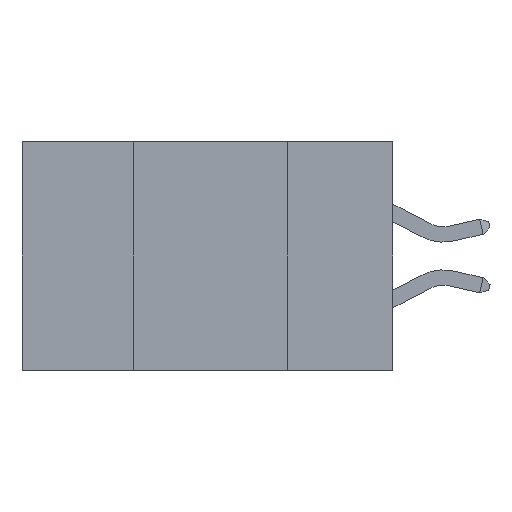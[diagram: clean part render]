
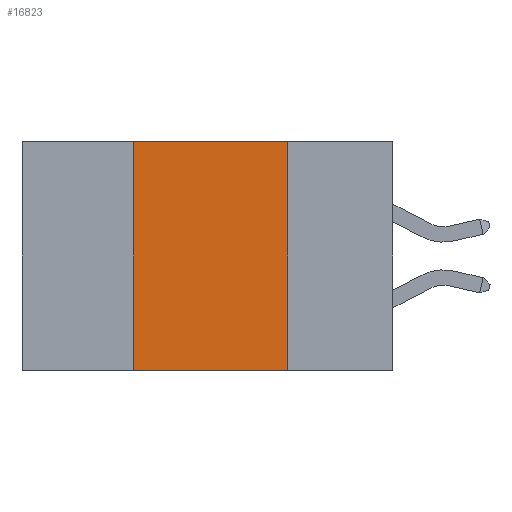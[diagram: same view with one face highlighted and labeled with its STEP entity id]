
A CAD part, left-side view. The second image highlights one B-rep face of the part: STEP entity #16823.
In plain terms, the highlighted planar face has unit normal (-1, 0, 0).
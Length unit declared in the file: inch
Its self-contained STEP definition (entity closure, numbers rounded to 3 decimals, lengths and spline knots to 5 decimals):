
#85 = EDGE_CURVE ( 'NONE', #16612, #15802, #24296, .T. ) ;
#560 = CARTESIAN_POINT ( 'NONE',  ( 0., 0.17, -0.37 ) ) ;
#592 = FACE_OUTER_BOUND ( 'NONE', #23139, .T. ) ;
#1837 = ORIENTED_EDGE ( 'NONE', *, *, #85, .F. ) ;
#2365 = CARTESIAN_POINT ( 'NONE',  ( 0., 0.42, 0. ) ) ;
#2491 = LINE ( 'NONE', #18236, #5283 ) ;
#3855 = CARTESIAN_POINT ( 'NONE',  ( 0., 0.42, -0.37 ) ) ;
#4566 = CARTESIAN_POINT ( 'NONE',  ( 0., 0.6, -0.37 ) ) ;
#5014 = AXIS2_PLACEMENT_3D ( 'NONE', #9945, #5709, #7823 ) ;
#5283 = VECTOR ( 'NONE', #9759, 39.37008 ) ;
#5709 = DIRECTION ( 'NONE',  ( 1., 0., 0. ) ) ;
#6066 = VERTEX_POINT ( 'NONE', #3855 ) ;
#6724 = DIRECTION ( 'NONE',  ( 0., 0., 1. ) ) ;
#7823 = DIRECTION ( 'NONE',  ( 0., 0., -1. ) ) ;
#8310 = EDGE_CURVE ( 'NONE', #6066, #16612, #23990, .T. ) ;
#8450 = DIRECTION ( 'NONE',  ( 0., -1., 0. ) ) ;
#9759 = DIRECTION ( 'NONE',  ( 0., 0., -1. ) ) ;
#9945 = CARTESIAN_POINT ( 'NONE',  ( 0., 0.6, 0. ) ) ;
#10954 = VERTEX_POINT ( 'NONE', #560 ) ;
#11721 = EDGE_CURVE ( 'NONE', #15802, #10954, #2491, .T. ) ;
#12038 = LINE ( 'NONE', #4566, #17434 ) ;
#14381 = CARTESIAN_POINT ( 'NONE',  ( 0., 0.17, 0. ) ) ;
#14513 = ORIENTED_EDGE ( 'NONE', *, *, #11721, .F. ) ;
#14798 = ORIENTED_EDGE ( 'NONE', *, *, #14904, .T. ) ;
#14904 = EDGE_CURVE ( 'NONE', #6066, #10954, #12038, .T. ) ;
#15802 = VERTEX_POINT ( 'NONE', #14381 ) ;
#16612 = VERTEX_POINT ( 'NONE', #19721 ) ;
#16823 = ADVANCED_FACE ( 'NONE', ( #592 ), #24073, .F. ) ;
#17090 = CARTESIAN_POINT ( 'NONE',  ( 0., 0.6, 0. ) ) ;
#17434 = VECTOR ( 'NONE', #8450, 39.37008 ) ;
#18236 = CARTESIAN_POINT ( 'NONE',  ( 0., 0.17, 0. ) ) ;
#19721 = CARTESIAN_POINT ( 'NONE',  ( 0., 0.42, 0. ) ) ;
#21169 = DIRECTION ( 'NONE',  ( 0., -1., 0. ) ) ;
#21780 = VECTOR ( 'NONE', #6724, 39.37008 ) ;
#23139 = EDGE_LOOP ( 'NONE', ( #14513, #1837, #23368, #14798 ) ) ;
#23368 = ORIENTED_EDGE ( 'NONE', *, *, #8310, .F. ) ;
#23990 = LINE ( 'NONE', #2365, #21780 ) ;
#24073 = PLANE ( 'NONE',  #5014 ) ;
#24296 = LINE ( 'NONE', #17090, #25894 ) ;
#25894 = VECTOR ( 'NONE', #21169, 39.37008 ) ;
